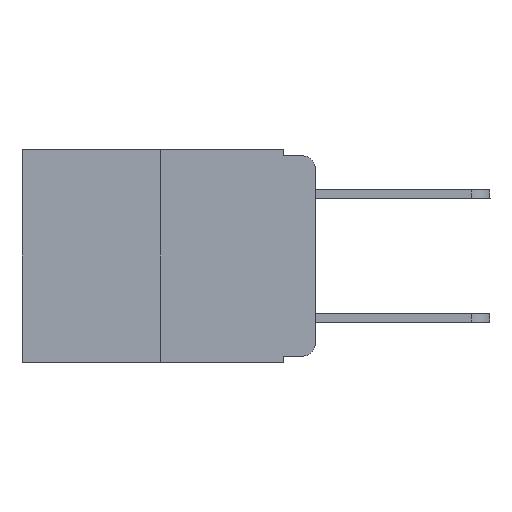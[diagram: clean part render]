
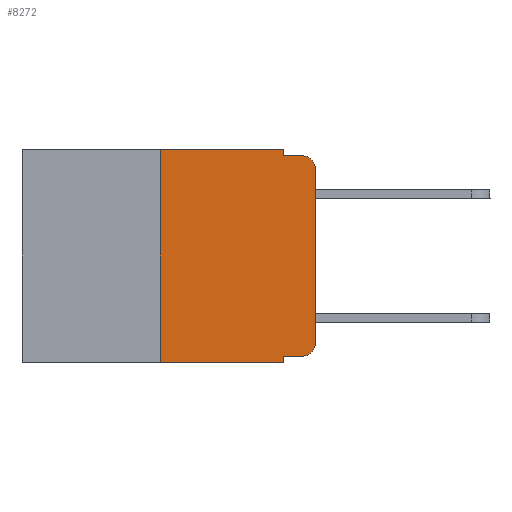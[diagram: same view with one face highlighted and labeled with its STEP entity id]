
A CAD part, left-side view. The second image highlights one B-rep face of the part: STEP entity #8272.
In plain terms, the highlighted planar face has unit normal (-1, 0, 0).
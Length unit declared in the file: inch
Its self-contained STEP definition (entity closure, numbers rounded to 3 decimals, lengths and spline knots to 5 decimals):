
#455 = CARTESIAN_POINT ( 'NONE',  ( 0., 0.051, 0. ) ) ;
#575 = DIRECTION ( 'NONE',  ( 0., 0., -1. ) ) ;
#1319 = VECTOR ( 'NONE', #4512, 39.37008 ) ;
#1357 = DIRECTION ( 'NONE',  ( 0., -1., 0. ) ) ;
#1433 = EDGE_CURVE ( 'NONE', #7897, #8609, #19472, .T. ) ;
#1482 = AXIS2_PLACEMENT_3D ( 'NONE', #22738, #20358, #18570 ) ;
#1658 = VECTOR ( 'NONE', #1357, 39.37008 ) ;
#2591 = VERTEX_POINT ( 'NONE', #4829 ) ;
#2778 = ORIENTED_EDGE ( 'NONE', *, *, #15174, .T. ) ;
#2933 = DIRECTION ( 'NONE',  ( 1., 0., 0. ) ) ;
#3619 = CARTESIAN_POINT ( 'NONE',  ( 0., 0.051, -0.333 ) ) ;
#3750 = DIRECTION ( 'NONE',  ( 0., -1., 0. ) ) ;
#4097 = ORIENTED_EDGE ( 'NONE', *, *, #12685, .F. ) ;
#4512 = DIRECTION ( 'NONE',  ( 0., 0., 1. ) ) ;
#4605 = PLANE ( 'NONE',  #18916 ) ;
#4609 = DIRECTION ( 'NONE',  ( 0., -1., 0. ) ) ;
#4626 = LINE ( 'NONE', #14060, #1319 ) ;
#4829 = CARTESIAN_POINT ( 'NONE',  ( 0., 0., -0.03 ) ) ;
#4936 = DIRECTION ( 'NONE',  ( 0., 0., -1. ) ) ;
#5273 = CARTESIAN_POINT ( 'NONE',  ( 0., 0.051, -0.01 ) ) ;
#5535 = VERTEX_POINT ( 'NONE', #5273 ) ;
#5749 = CARTESIAN_POINT ( 'NONE',  ( 0., 0.25, -0.343 ) ) ;
#5767 = VERTEX_POINT ( 'NONE', #5749 ) ;
#6472 = EDGE_CURVE ( 'NONE', #5767, #17978, #4626, .T. ) ;
#6733 = LINE ( 'NONE', #21305, #8357 ) ;
#6761 = DIRECTION ( 'NONE',  ( 0., -1., 0. ) ) ;
#7336 = LINE ( 'NONE', #12696, #7750 ) ;
#7750 = VECTOR ( 'NONE', #3750, 39.37008 ) ;
#7897 = VERTEX_POINT ( 'NONE', #10722 ) ;
#8272 = ADVANCED_FACE ( 'NONE', ( #13692 ), #4605, .F. ) ;
#8357 = VECTOR ( 'NONE', #4936, 39.37008 ) ;
#8609 = VERTEX_POINT ( 'NONE', #11758 ) ;
#8635 = LINE ( 'NONE', #12215, #1658 ) ;
#8756 = VECTOR ( 'NONE', #12521, 39.37008 ) ;
#8816 = ORIENTED_EDGE ( 'NONE', *, *, #6472, .F. ) ;
#9191 = AXIS2_PLACEMENT_3D ( 'NONE', #22691, #10044, #15287 ) ;
#9514 = LINE ( 'NONE', #455, #19813 ) ;
#9624 = EDGE_CURVE ( 'NONE', #18718, #7897, #15938, .T. ) ;
#9778 = VERTEX_POINT ( 'NONE', #12714 ) ;
#9993 = CARTESIAN_POINT ( 'NONE',  ( 0., 0.473, 0. ) ) ;
#10044 = DIRECTION ( 'NONE',  ( -1., 0., 0. ) ) ;
#10458 = DIRECTION ( 'NONE',  ( 0., 0., -1. ) ) ;
#10624 = LINE ( 'NONE', #21599, #8756 ) ;
#10649 = ORIENTED_EDGE ( 'NONE', *, *, #14221, .F. ) ;
#10722 = CARTESIAN_POINT ( 'NONE',  ( 0., 0.02, -0.333 ) ) ;
#11213 = ORIENTED_EDGE ( 'NONE', *, *, #22090, .F. ) ;
#11623 = ORIENTED_EDGE ( 'NONE', *, *, #20429, .T. ) ;
#11758 = CARTESIAN_POINT ( 'NONE',  ( 0., 0., -0.313 ) ) ;
#11817 = ORIENTED_EDGE ( 'NONE', *, *, #1433, .T. ) ;
#11905 = ORIENTED_EDGE ( 'NONE', *, *, #9624, .T. ) ;
#12215 = CARTESIAN_POINT ( 'NONE',  ( 0., 0.051, -0.01 ) ) ;
#12521 = DIRECTION ( 'NONE',  ( 0., 0., 1. ) ) ;
#12685 = EDGE_CURVE ( 'NONE', #17978, #22122, #15709, .T. ) ;
#12696 = CARTESIAN_POINT ( 'NONE',  ( 0., 0.473, -0.343 ) ) ;
#12714 = CARTESIAN_POINT ( 'NONE',  ( 0., 0.051, -0.343 ) ) ;
#12858 = VECTOR ( 'NONE', #6761, 39.37008 ) ;
#13692 = FACE_OUTER_BOUND ( 'NONE', #15158, .T. ) ;
#14060 = CARTESIAN_POINT ( 'NONE',  ( 0., 0.25, 0. ) ) ;
#14095 = EDGE_CURVE ( 'NONE', #2591, #15200, #14432, .T. ) ;
#14221 = EDGE_CURVE ( 'NONE', #22122, #5535, #6733, .T. ) ;
#14432 = CIRCLE ( 'NONE', #1482, 0.02 ) ;
#15158 = EDGE_LOOP ( 'NONE', ( #2778, #20212, #11213, #10649, #4097, #8816, #11623, #15634, #11905, #11817 ) ) ;
#15174 = EDGE_CURVE ( 'NONE', #8609, #2591, #10624, .T. ) ;
#15200 = VERTEX_POINT ( 'NONE', #17997 ) ;
#15287 = DIRECTION ( 'NONE',  ( 0., 0., -1. ) ) ;
#15634 = ORIENTED_EDGE ( 'NONE', *, *, #17157, .F. ) ;
#15709 = LINE ( 'NONE', #21215, #12858 ) ;
#15938 = LINE ( 'NONE', #19635, #21587 ) ;
#17157 = EDGE_CURVE ( 'NONE', #18718, #9778, #9514, .T. ) ;
#17924 = CARTESIAN_POINT ( 'NONE',  ( 0., 0.051, 0. ) ) ;
#17978 = VERTEX_POINT ( 'NONE', #20405 ) ;
#17997 = CARTESIAN_POINT ( 'NONE',  ( 0., 0.02, -0.01 ) ) ;
#18570 = DIRECTION ( 'NONE',  ( 0., 0., -1. ) ) ;
#18718 = VERTEX_POINT ( 'NONE', #3619 ) ;
#18916 = AXIS2_PLACEMENT_3D ( 'NONE', #9993, #2933, #10458 ) ;
#19472 = CIRCLE ( 'NONE', #9191, 0.02 ) ;
#19635 = CARTESIAN_POINT ( 'NONE',  ( 0., 0.051, -0.333 ) ) ;
#19813 = VECTOR ( 'NONE', #575, 39.37008 ) ;
#20212 = ORIENTED_EDGE ( 'NONE', *, *, #14095, .T. ) ;
#20358 = DIRECTION ( 'NONE',  ( -1., 0., 0. ) ) ;
#20405 = CARTESIAN_POINT ( 'NONE',  ( 0., 0.25, 0. ) ) ;
#20429 = EDGE_CURVE ( 'NONE', #5767, #9778, #7336, .T. ) ;
#21215 = CARTESIAN_POINT ( 'NONE',  ( 0., 0.473, 0. ) ) ;
#21305 = CARTESIAN_POINT ( 'NONE',  ( 0., 0.051, 0. ) ) ;
#21587 = VECTOR ( 'NONE', #4609, 39.37008 ) ;
#21599 = CARTESIAN_POINT ( 'NONE',  ( 0., 0., 0. ) ) ;
#22090 = EDGE_CURVE ( 'NONE', #5535, #15200, #8635, .T. ) ;
#22122 = VERTEX_POINT ( 'NONE', #17924 ) ;
#22691 = CARTESIAN_POINT ( 'NONE',  ( 0., 0.02, -0.313 ) ) ;
#22738 = CARTESIAN_POINT ( 'NONE',  ( 0., 0.02, -0.03 ) ) ;
